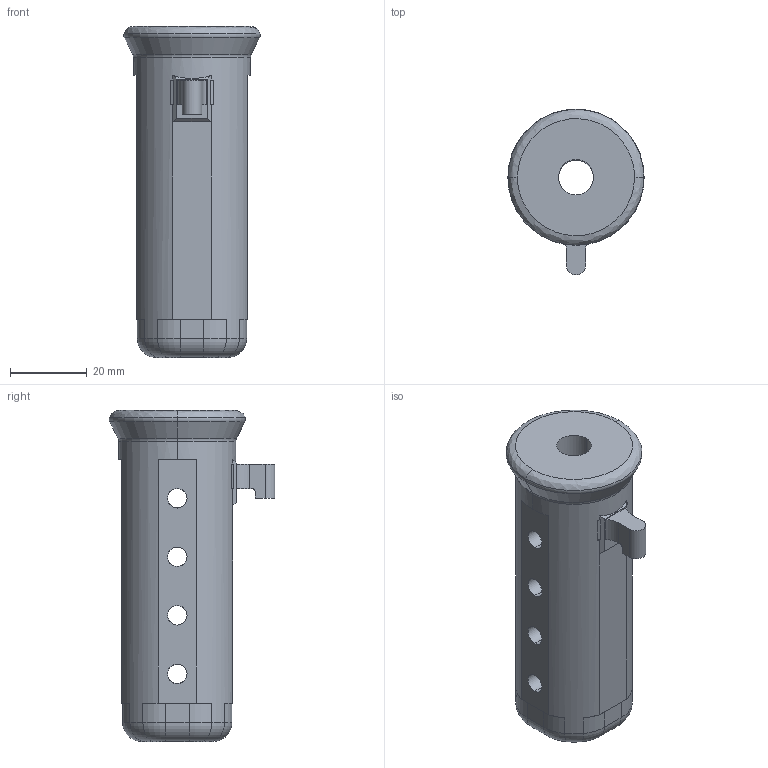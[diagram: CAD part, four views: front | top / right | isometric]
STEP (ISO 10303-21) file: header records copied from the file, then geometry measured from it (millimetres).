
FILE_DESCRIPTION (( 'STEP AP214' ), '1' );
FILE_NAME ('ventedbarrel.STEP', '2013-07-04T02:37:46', ( '' ), ( '' ), 'SwSTEP 2.0', 'SolidWorks 2012', '' );
FILE_SCHEMA (( 'AUTOMOTIVE_DESIGN' ));
Length unit declared in the file: millimetre
Products named in the file (1): ventedbarrel
Bounding box: 35.48 x 43.14 x 86.2 mm (x, y, z)
Volume: 54153.1 mm3; surface area: 13736.6 mm2
Topology: 1 solids, 1 shells, 102 faces, 276 edges, 169 vertices
Faces by surface type: cylinder 47, plane 31, torus 20, bspline 2, cone 2
Entity records: 3974 total; most frequent: CARTESIAN_POINT 1297, DIRECTION 577, ORIENTED_EDGE 552, EDGE_CURVE 276, AXIS2_PLACEMENT_3D 229, VERTEX_POINT 169, CIRCLE 128, EDGE_LOOP 121
